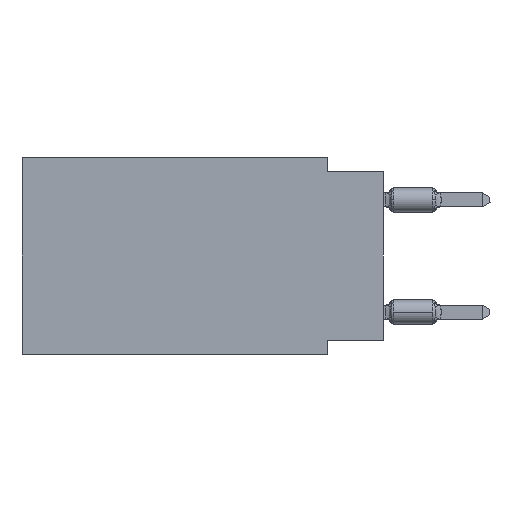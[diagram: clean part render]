
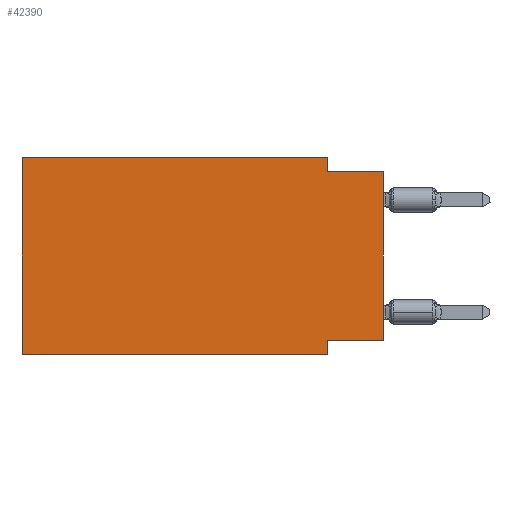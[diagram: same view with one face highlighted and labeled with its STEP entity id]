
A CAD part, left-side view. The second image highlights one B-rep face of the part: STEP entity #42390.
In plain terms, the highlighted planar face has unit normal (-1, 0, 0).
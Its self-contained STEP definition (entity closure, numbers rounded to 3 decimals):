
#854 = EDGE_CURVE ( 'NONE', #23474, #2858, #63460, .T. ) ;
#1338 = VECTOR ( 'NONE', #46810, 1000. ) ;
#2334 = LINE ( 'NONE', #53360, #1338 ) ;
#2691 = CARTESIAN_POINT ( 'NONE',  ( 0., 16.383, 0. ) ) ;
#2858 = VERTEX_POINT ( 'NONE', #52906 ) ;
#2881 = ORIENTED_EDGE ( 'NONE', *, *, #24196, .F. ) ;
#3566 = CARTESIAN_POINT ( 'NONE',  ( 0., 2.54, -8.89 ) ) ;
#6750 = LINE ( 'NONE', #58128, #62884 ) ;
#9058 = CARTESIAN_POINT ( 'NONE',  ( 0., 0., -0.635 ) ) ;
#9157 = EDGE_LOOP ( 'NONE', ( #62813, #35562, #45952, #17491, #16524, #57171, #17819, #2881 ) ) ;
#10363 = VECTOR ( 'NONE', #71426, 1000. ) ;
#10886 = CARTESIAN_POINT ( 'NONE',  ( 0., 16.383, 0. ) ) ;
#11256 = LINE ( 'NONE', #10886, #10363 ) ;
#11438 = EDGE_CURVE ( 'NONE', #24240, #62243, #19257, .T. ) ;
#13516 = DIRECTION ( 'NONE',  ( 0., 0., -1. ) ) ;
#15959 = VECTOR ( 'NONE', #58455, 1000. ) ;
#16524 = ORIENTED_EDGE ( 'NONE', *, *, #45205, .F. ) ;
#16535 = PLANE ( 'NONE',  #50003 ) ;
#17491 = ORIENTED_EDGE ( 'NONE', *, *, #25458, .F. ) ;
#17819 = ORIENTED_EDGE ( 'NONE', *, *, #11438, .F. ) ;
#19257 = LINE ( 'NONE', #3566, #26612 ) ;
#23474 = VERTEX_POINT ( 'NONE', #62834 ) ;
#24196 = EDGE_CURVE ( 'NONE', #42698, #24240, #57530, .T. ) ;
#24240 = VERTEX_POINT ( 'NONE', #25792 ) ;
#25458 = EDGE_CURVE ( 'NONE', #42425, #23474, #11256, .T. ) ;
#25792 = CARTESIAN_POINT ( 'NONE',  ( 0., 2.54, -8.255 ) ) ;
#26612 = VECTOR ( 'NONE', #41520, 1000. ) ;
#26900 = VECTOR ( 'NONE', #13516, 1000. ) ;
#28632 = VERTEX_POINT ( 'NONE', #29787 ) ;
#29787 = CARTESIAN_POINT ( 'NONE',  ( 0., 16.383, -8.89 ) ) ;
#34611 = CARTESIAN_POINT ( 'NONE',  ( 0., 0., -8.255 ) ) ;
#35299 = VECTOR ( 'NONE', #68472, 1000. ) ;
#35562 = ORIENTED_EDGE ( 'NONE', *, *, #38776, .F. ) ;
#37457 = DIRECTION ( 'NONE',  ( 1., 0., 0. ) ) ;
#38597 = CARTESIAN_POINT ( 'NONE',  ( 0., 0., 0. ) ) ;
#38776 = EDGE_CURVE ( 'NONE', #2858, #47169, #6750, .T. ) ;
#38796 = CARTESIAN_POINT ( 'NONE',  ( 0., 16.383, 0. ) ) ;
#39230 = EDGE_CURVE ( 'NONE', #42698, #47169, #66642, .T. ) ;
#40130 = DIRECTION ( 'NONE',  ( 0., -1., 0. ) ) ;
#40406 = CARTESIAN_POINT ( 'NONE',  ( 0., 2.54, -8.89 ) ) ;
#41520 = DIRECTION ( 'NONE',  ( 0., 0., -1. ) ) ;
#41591 = CARTESIAN_POINT ( 'NONE',  ( 0., 2.54, 0. ) ) ;
#42390 = ADVANCED_FACE ( 'NONE', ( #66851 ), #16535, .F. ) ;
#42425 = VERTEX_POINT ( 'NONE', #53842 ) ;
#42698 = VERTEX_POINT ( 'NONE', #55277 ) ;
#45205 = EDGE_CURVE ( 'NONE', #28632, #42425, #48606, .T. ) ;
#45952 = ORIENTED_EDGE ( 'NONE', *, *, #854, .F. ) ;
#46634 = VECTOR ( 'NONE', #49902, 1000. ) ;
#46810 = DIRECTION ( 'NONE',  ( 0., -1., 0. ) ) ;
#47169 = VERTEX_POINT ( 'NONE', #9058 ) ;
#48606 = LINE ( 'NONE', #2691, #15959 ) ;
#49902 = DIRECTION ( 'NONE',  ( 0., 0., 1. ) ) ;
#50003 = AXIS2_PLACEMENT_3D ( 'NONE', #38796, #37457, #69884 ) ;
#52906 = CARTESIAN_POINT ( 'NONE',  ( 0., 2.54, -0.635 ) ) ;
#53360 = CARTESIAN_POINT ( 'NONE',  ( 0., 16.383, -8.89 ) ) ;
#53775 = EDGE_CURVE ( 'NONE', #28632, #62243, #2334, .T. ) ;
#53842 = CARTESIAN_POINT ( 'NONE',  ( 0., 16.383, 0. ) ) ;
#55277 = CARTESIAN_POINT ( 'NONE',  ( 0., 0., -8.255 ) ) ;
#57171 = ORIENTED_EDGE ( 'NONE', *, *, #53775, .T. ) ;
#57530 = LINE ( 'NONE', #34611, #35299 ) ;
#58128 = CARTESIAN_POINT ( 'NONE',  ( 0., 0., -0.635 ) ) ;
#58455 = DIRECTION ( 'NONE',  ( 0., 0., 1. ) ) ;
#62243 = VERTEX_POINT ( 'NONE', #40406 ) ;
#62813 = ORIENTED_EDGE ( 'NONE', *, *, #39230, .T. ) ;
#62834 = CARTESIAN_POINT ( 'NONE',  ( 0., 2.54, 0. ) ) ;
#62884 = VECTOR ( 'NONE', #40130, 1000. ) ;
#63460 = LINE ( 'NONE', #41591, #26900 ) ;
#66642 = LINE ( 'NONE', #38597, #46634 ) ;
#66851 = FACE_OUTER_BOUND ( 'NONE', #9157, .T. ) ;
#68472 = DIRECTION ( 'NONE',  ( 0., 1., 0. ) ) ;
#69884 = DIRECTION ( 'NONE',  ( 0., 0., -1. ) ) ;
#71426 = DIRECTION ( 'NONE',  ( 0., -1., 0. ) ) ;
